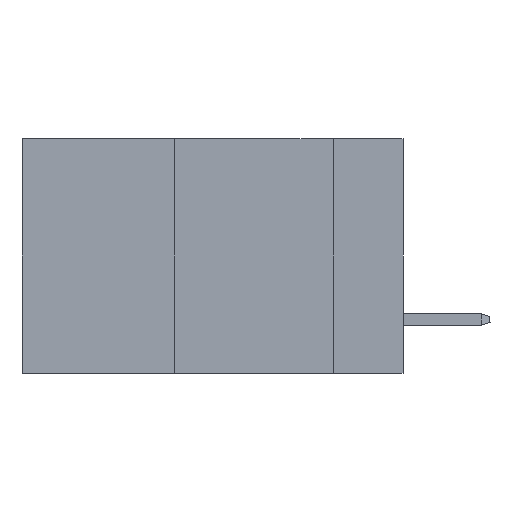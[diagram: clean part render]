
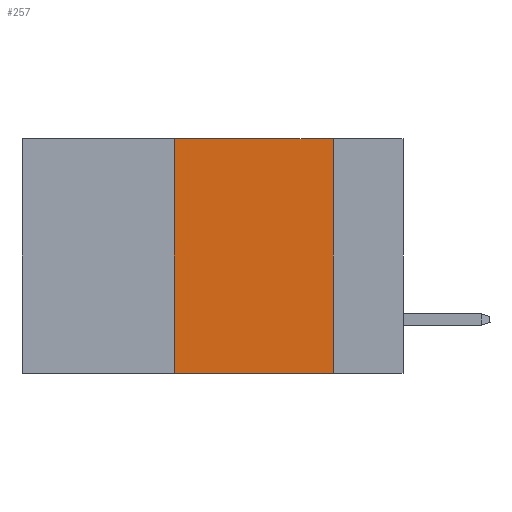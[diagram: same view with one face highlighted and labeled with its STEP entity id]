
A CAD part, left-side view. The second image highlights one B-rep face of the part: STEP entity #257.
In plain terms, the highlighted planar face has unit normal (-1, 0, 0).
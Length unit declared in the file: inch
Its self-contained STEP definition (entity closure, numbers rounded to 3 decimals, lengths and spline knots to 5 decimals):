
#257 = ADVANCED_FACE ( 'NONE', ( #37064 ), #3880, .F. ) ;
#1634 = LINE ( 'NONE', #42057, #8600 ) ;
#2658 = LINE ( 'NONE', #29479, #19754 ) ;
#2836 = VECTOR ( 'NONE', #10610, 39.37008 ) ;
#2936 = ORIENTED_EDGE ( 'NONE', *, *, #38190, .T. ) ;
#3042 = VERTEX_POINT ( 'NONE', #16012 ) ;
#3577 = VERTEX_POINT ( 'NONE', #5525 ) ;
#3880 = PLANE ( 'NONE',  #4101 ) ;
#4101 = AXIS2_PLACEMENT_3D ( 'NONE', #22027, #15502, #44534 ) ;
#5525 = CARTESIAN_POINT ( 'NONE',  ( 0., 0.36, -0.37 ) ) ;
#7452 = LINE ( 'NONE', #10356, #2836 ) ;
#7948 = CARTESIAN_POINT ( 'NONE',  ( 0., 0.11, 0. ) ) ;
#8600 = VECTOR ( 'NONE', #31869, 39.37008 ) ;
#10356 = CARTESIAN_POINT ( 'NONE',  ( 0., 0.11, 0. ) ) ;
#10610 = DIRECTION ( 'NONE',  ( 0., 0., -1. ) ) ;
#11103 = VERTEX_POINT ( 'NONE', #17048 ) ;
#11953 = CARTESIAN_POINT ( 'NONE',  ( 0., 0.36, 0. ) ) ;
#12989 = VECTOR ( 'NONE', #26952, 39.37008 ) ;
#14540 = VERTEX_POINT ( 'NONE', #7948 ) ;
#15502 = DIRECTION ( 'NONE',  ( 1., 0., 0. ) ) ;
#16012 = CARTESIAN_POINT ( 'NONE',  ( 0., 0.11, -0.37 ) ) ;
#16134 = EDGE_CURVE ( 'NONE', #11103, #14540, #2658, .T. ) ;
#16537 = LINE ( 'NONE', #11953, #12989 ) ;
#17048 = CARTESIAN_POINT ( 'NONE',  ( 0., 0.36, 0. ) ) ;
#19754 = VECTOR ( 'NONE', #43342, 39.37008 ) ;
#22027 = CARTESIAN_POINT ( 'NONE',  ( 0., 0.6, 0. ) ) ;
#24176 = EDGE_CURVE ( 'NONE', #3577, #11103, #16537, .T. ) ;
#26952 = DIRECTION ( 'NONE',  ( 0., 0., 1. ) ) ;
#27167 = ORIENTED_EDGE ( 'NONE', *, *, #24176, .F. ) ;
#29479 = CARTESIAN_POINT ( 'NONE',  ( 0., 0.6, 0. ) ) ;
#31869 = DIRECTION ( 'NONE',  ( 0., -1., 0. ) ) ;
#37064 = FACE_OUTER_BOUND ( 'NONE', #45635, .T. ) ;
#38190 = EDGE_CURVE ( 'NONE', #3577, #3042, #1634, .T. ) ;
#42057 = CARTESIAN_POINT ( 'NONE',  ( 0., 0.6, -0.37 ) ) ;
#43342 = DIRECTION ( 'NONE',  ( 0., -1., 0. ) ) ;
#43921 = ORIENTED_EDGE ( 'NONE', *, *, #16134, .F. ) ;
#44470 = ORIENTED_EDGE ( 'NONE', *, *, #45320, .F. ) ;
#44534 = DIRECTION ( 'NONE',  ( 0., 0., -1. ) ) ;
#45320 = EDGE_CURVE ( 'NONE', #14540, #3042, #7452, .T. ) ;
#45635 = EDGE_LOOP ( 'NONE', ( #44470, #43921, #27167, #2936 ) ) ;
